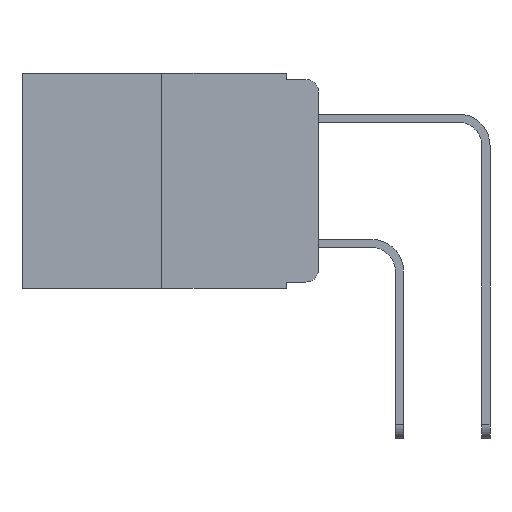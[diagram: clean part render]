
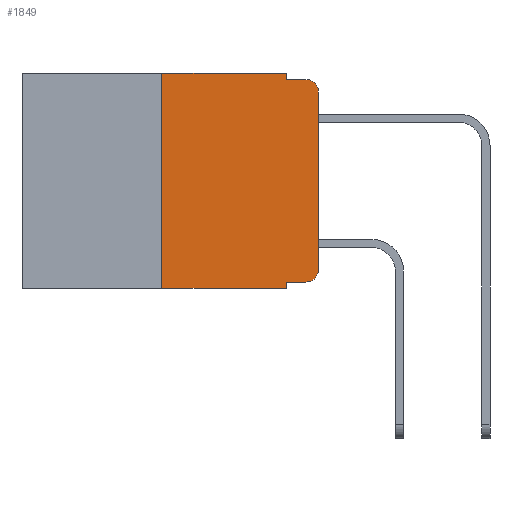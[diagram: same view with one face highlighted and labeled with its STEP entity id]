
A CAD part, left-side view. The second image highlights one B-rep face of the part: STEP entity #1849.
In plain terms, the highlighted planar face has unit normal (-1, 0, 0).
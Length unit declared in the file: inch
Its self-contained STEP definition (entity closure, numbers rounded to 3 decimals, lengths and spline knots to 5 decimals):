
#24 = VERTEX_POINT ( 'NONE', #11525 ) ;
#70 = LINE ( 'NONE', #8929, #10254 ) ;
#347 = VERTEX_POINT ( 'NONE', #1236 ) ;
#490 = DIRECTION ( 'NONE',  ( 0., 0., -1. ) ) ;
#493 = CARTESIAN_POINT ( 'NONE',  ( 0., 0.02, -0.313 ) ) ;
#762 = DIRECTION ( 'NONE',  ( 0., -1., 0. ) ) ;
#960 = VECTOR ( 'NONE', #4530, 39.37008 ) ;
#1227 = DIRECTION ( 'NONE',  ( 0., 0., 1. ) ) ;
#1236 = CARTESIAN_POINT ( 'NONE',  ( 0., 0., -0.03 ) ) ;
#1441 = VERTEX_POINT ( 'NONE', #12827 ) ;
#1464 = LINE ( 'NONE', #11821, #11848 ) ;
#1532 = DIRECTION ( 'NONE',  ( 0., 0., -1. ) ) ;
#1653 = VECTOR ( 'NONE', #9391, 39.37008 ) ;
#1849 = ADVANCED_FACE ( 'NONE', ( #2321 ), #8859, .F. ) ;
#1872 = CARTESIAN_POINT ( 'NONE',  ( 0., 0.473, 0. ) ) ;
#1884 = EDGE_CURVE ( 'NONE', #5381, #11320, #4409, .T. ) ;
#2074 = ORIENTED_EDGE ( 'NONE', *, *, #6350, .F. ) ;
#2163 = AXIS2_PLACEMENT_3D ( 'NONE', #9362, #10747, #10631 ) ;
#2321 = FACE_OUTER_BOUND ( 'NONE', #8444, .T. ) ;
#2390 = ORIENTED_EDGE ( 'NONE', *, *, #12723, .T. ) ;
#2553 = VERTEX_POINT ( 'NONE', #5389 ) ;
#2867 = ORIENTED_EDGE ( 'NONE', *, *, #1884, .F. ) ;
#2869 = VERTEX_POINT ( 'NONE', #11246 ) ;
#3561 = CIRCLE ( 'NONE', #8277, 0.02 ) ;
#3943 = LINE ( 'NONE', #12965, #11599 ) ;
#4011 = VECTOR ( 'NONE', #762, 39.37008 ) ;
#4372 = LINE ( 'NONE', #9168, #12000 ) ;
#4409 = LINE ( 'NONE', #10586, #1653 ) ;
#4530 = DIRECTION ( 'NONE',  ( 0., 0., -1. ) ) ;
#4654 = LINE ( 'NONE', #7889, #4011 ) ;
#4707 = LINE ( 'NONE', #1872, #10673 ) ;
#4770 = EDGE_CURVE ( 'NONE', #2553, #2869, #70, .T. ) ;
#5048 = CARTESIAN_POINT ( 'NONE',  ( 0., 0.051, -0.01 ) ) ;
#5381 = VERTEX_POINT ( 'NONE', #8117 ) ;
#5389 = CARTESIAN_POINT ( 'NONE',  ( 0., 0.25, -0.343 ) ) ;
#6350 = EDGE_CURVE ( 'NONE', #8161, #5381, #4707, .T. ) ;
#6356 = CIRCLE ( 'NONE', #6731, 0.02 ) ;
#6448 = LINE ( 'NONE', #7544, #960 ) ;
#6642 = DIRECTION ( 'NONE',  ( -1., 0., 0. ) ) ;
#6731 = AXIS2_PLACEMENT_3D ( 'NONE', #493, #7663, #1532 ) ;
#6837 = EDGE_CURVE ( 'NONE', #24, #347, #4372, .T. ) ;
#7508 = ORIENTED_EDGE ( 'NONE', *, *, #12100, .F. ) ;
#7544 = CARTESIAN_POINT ( 'NONE',  ( 0., 0.051, 0. ) ) ;
#7663 = DIRECTION ( 'NONE',  ( -1., 0., 0. ) ) ;
#7826 = ORIENTED_EDGE ( 'NONE', *, *, #8224, .T. ) ;
#7889 = CARTESIAN_POINT ( 'NONE',  ( 0., 0.051, -0.333 ) ) ;
#7967 = ORIENTED_EDGE ( 'NONE', *, *, #6837, .T. ) ;
#8117 = CARTESIAN_POINT ( 'NONE',  ( 0., 0.051, 0. ) ) ;
#8141 = ORIENTED_EDGE ( 'NONE', *, *, #11198, .F. ) ;
#8161 = VERTEX_POINT ( 'NONE', #11993 ) ;
#8224 = EDGE_CURVE ( 'NONE', #10069, #1441, #4654, .T. ) ;
#8277 = AXIS2_PLACEMENT_3D ( 'NONE', #12504, #6642, #490 ) ;
#8361 = DIRECTION ( 'NONE',  ( 0., -1., 0. ) ) ;
#8444 = EDGE_LOOP ( 'NONE', ( #7967, #2390, #12249, #2867, #2074, #8141, #9050, #7508, #7826, #8460 ) ) ;
#8460 = ORIENTED_EDGE ( 'NONE', *, *, #9242, .T. ) ;
#8856 = CARTESIAN_POINT ( 'NONE',  ( 0., 0.051, -0.333 ) ) ;
#8859 = PLANE ( 'NONE',  #2163 ) ;
#8906 = DIRECTION ( 'NONE',  ( 0., 0., 1. ) ) ;
#8929 = CARTESIAN_POINT ( 'NONE',  ( 0., 0.473, -0.343 ) ) ;
#9050 = ORIENTED_EDGE ( 'NONE', *, *, #4770, .T. ) ;
#9168 = CARTESIAN_POINT ( 'NONE',  ( 0., 0., 0. ) ) ;
#9242 = EDGE_CURVE ( 'NONE', #1441, #24, #6356, .T. ) ;
#9339 = DIRECTION ( 'NONE',  ( 0., -1., 0. ) ) ;
#9362 = CARTESIAN_POINT ( 'NONE',  ( 0., 0.473, 0. ) ) ;
#9391 = DIRECTION ( 'NONE',  ( 0., 0., -1. ) ) ;
#9639 = EDGE_CURVE ( 'NONE', #11320, #10956, #3943, .T. ) ;
#10069 = VERTEX_POINT ( 'NONE', #8856 ) ;
#10254 = VECTOR ( 'NONE', #8361, 39.37008 ) ;
#10586 = CARTESIAN_POINT ( 'NONE',  ( 0., 0.051, 0. ) ) ;
#10631 = DIRECTION ( 'NONE',  ( 0., 0., -1. ) ) ;
#10673 = VECTOR ( 'NONE', #9339, 39.37008 ) ;
#10747 = DIRECTION ( 'NONE',  ( 1., 0., 0. ) ) ;
#10956 = VERTEX_POINT ( 'NONE', #12358 ) ;
#11198 = EDGE_CURVE ( 'NONE', #2553, #8161, #1464, .T. ) ;
#11246 = CARTESIAN_POINT ( 'NONE',  ( 0., 0.051, -0.343 ) ) ;
#11320 = VERTEX_POINT ( 'NONE', #5048 ) ;
#11525 = CARTESIAN_POINT ( 'NONE',  ( 0., 0., -0.313 ) ) ;
#11599 = VECTOR ( 'NONE', #12070, 39.37008 ) ;
#11821 = CARTESIAN_POINT ( 'NONE',  ( 0., 0.25, 0. ) ) ;
#11848 = VECTOR ( 'NONE', #8906, 39.37008 ) ;
#11993 = CARTESIAN_POINT ( 'NONE',  ( 0., 0.25, 0. ) ) ;
#12000 = VECTOR ( 'NONE', #1227, 39.37008 ) ;
#12070 = DIRECTION ( 'NONE',  ( 0., -1., 0. ) ) ;
#12100 = EDGE_CURVE ( 'NONE', #10069, #2869, #6448, .T. ) ;
#12249 = ORIENTED_EDGE ( 'NONE', *, *, #9639, .F. ) ;
#12358 = CARTESIAN_POINT ( 'NONE',  ( 0., 0.02, -0.01 ) ) ;
#12504 = CARTESIAN_POINT ( 'NONE',  ( 0., 0.02, -0.03 ) ) ;
#12723 = EDGE_CURVE ( 'NONE', #347, #10956, #3561, .T. ) ;
#12827 = CARTESIAN_POINT ( 'NONE',  ( 0., 0.02, -0.333 ) ) ;
#12965 = CARTESIAN_POINT ( 'NONE',  ( 0., 0.051, -0.01 ) ) ;
